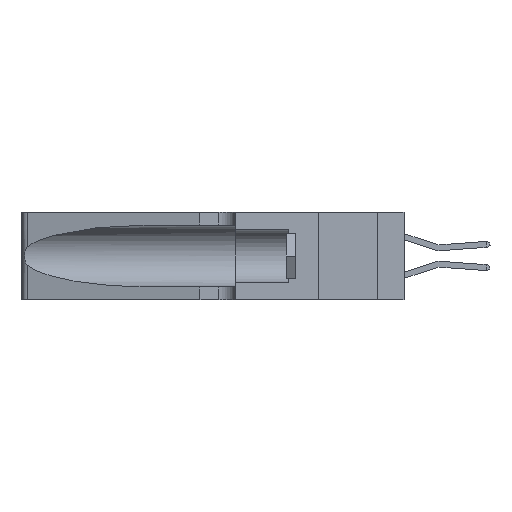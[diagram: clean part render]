
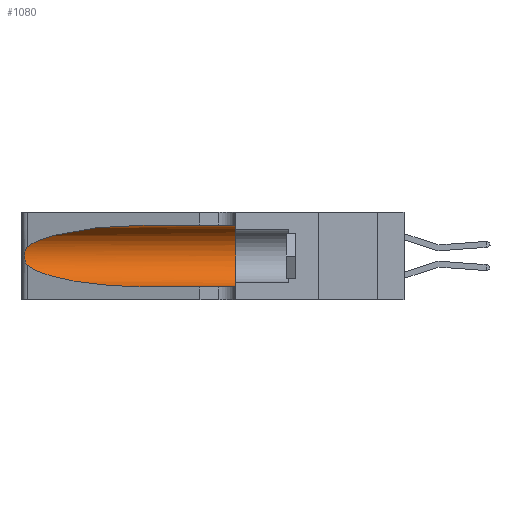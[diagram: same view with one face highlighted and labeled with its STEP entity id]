
A CAD part, left-side view. The second image highlights one B-rep face of the part: STEP entity #1080.
In plain terms, the highlighted cylindrical face has radius 3.308 mm (diameter 6.617 mm), a partial arc.
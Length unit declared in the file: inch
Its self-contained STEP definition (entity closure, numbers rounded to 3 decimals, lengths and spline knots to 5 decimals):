
#271 = CARTESIAN_POINT ( 'NONE',  ( 0.1305, 1.61858, 0.05475 ) ) ;
#1080 = ADVANCED_FACE ( 'NONE', ( #2937 ), #16985, .F. ) ;
#2819 = CARTESIAN_POINT ( 'NONE',  ( 0.25789, 1.23486, 0.15765 ) ) ;
#2937 = FACE_OUTER_BOUND ( 'NONE', #26758, .T. ) ;
#3029 = LINE ( 'NONE', #271, #32504 ) ;
#3994 = CARTESIAN_POINT ( 'NONE',  ( 0.1305, 0.72297, 0.31525 ) ) ;
#4893 = CARTESIAN_POINT ( 'NONE',  ( 0.1305, 0.72297, 0.31525 ) ) ;
#5700 = CARTESIAN_POINT ( 'NONE',  ( 0.25555, 1.22993, 0.14849 ) ) ;
#6794 = EDGE_CURVE ( 'NONE', #8950, #34060, #3029, .T. ) ;
#8090 = AXIS2_PLACEMENT_3D ( 'NONE', #16052, #35247, #18806 ) ;
#8423 = CARTESIAN_POINT ( 'NONE',  ( 0.25555, 1.22994, 0.2215 ) ) ;
#8950 = VERTEX_POINT ( 'NONE', #14795 ) ;
#9006 = CARTESIAN_POINT ( 'NONE',  ( 0.25487, 1.22718, 0.14631 ) ) ;
#9225 =( BOUNDED_CURVE ( )  B_SPLINE_CURVE ( 3, ( #4893, #10586, #32580, #16168 ),
 .UNSPECIFIED., .F., .F. ) 
 B_SPLINE_CURVE_WITH_KNOTS ( ( 4, 4 ),
 ( 1.5708, 2.84003 ),
 .UNSPECIFIED. ) 
 CURVE ( )  GEOMETRIC_REPRESENTATION_ITEM ( )  RATIONAL_B_SPLINE_CURVE ( ( 1., 0.87, 0.87, 1. ) ) 
 REPRESENTATION_ITEM ( '' )  );
#9390 = EDGE_CURVE ( 'NONE', #27486, #15746, #28443, .T. ) ;
#10586 = CARTESIAN_POINT ( 'NONE',  ( 0.18966, 0.96281, 0.31525 ) ) ;
#10595 = CARTESIAN_POINT ( 'NONE',  ( 0.18966, 0.96281, 0.05475 ) ) ;
#10683 = VECTOR ( 'NONE', #17556, 39.37008 ) ;
#11247 = CARTESIAN_POINT ( 'NONE',  ( 0.25787, 1.23484, 0.2124 ) ) ;
#12180 = ORIENTED_EDGE ( 'NONE', *, *, #18958, .T. ) ;
#14048 = CARTESIAN_POINT ( 'NONE',  ( 0.26018, 1.23835, 0.19895 ) ) ;
#14157 = CARTESIAN_POINT ( 'NONE',  ( 0.25487, 1.22718, 0.22369 ) ) ;
#14790 = CARTESIAN_POINT ( 'NONE',  ( 0.1305, 1.61858, 0.31525 ) ) ;
#14795 = CARTESIAN_POINT ( 'NONE',  ( 0.1305, 0.72297, 0.05475 ) ) ;
#15037 = CIRCLE ( 'NONE', #8090, 0.13025 ) ;
#15645 = ORIENTED_EDGE ( 'NONE', *, *, #28571, .T. ) ;
#15746 = VERTEX_POINT ( 'NONE', #9006 ) ;
#16052 = CARTESIAN_POINT ( 'NONE',  ( 0.1305, 0.35, 0.185 ) ) ;
#16168 = CARTESIAN_POINT ( 'NONE',  ( 0.25487, 1.22718, 0.22369 ) ) ;
#16812 = CARTESIAN_POINT ( 'NONE',  ( 0.26075, 1.23896, 0.178 ) ) ;
#16985 = CYLINDRICAL_SURFACE ( 'NONE', #23046, 0.13025 ) ;
#17556 = DIRECTION ( 'NONE',  ( 0., -1., 0. ) ) ;
#18230 = ORIENTED_EDGE ( 'NONE', *, *, #35185, .F. ) ;
#18806 = DIRECTION ( 'NONE',  ( 0., 0., 1. ) ) ;
#18958 = EDGE_CURVE ( 'NONE', #34624, #27486, #9225, .T. ) ;
#19579 = CARTESIAN_POINT ( 'NONE',  ( 0.25856, 1.23593, 0.16098 ) ) ;
#19929 = DIRECTION ( 'NONE',  ( 0., -1., 0. ) ) ;
#21057 = CARTESIAN_POINT ( 'NONE',  ( 0.1305, 0.35, 0.31525 ) ) ;
#22330 = CARTESIAN_POINT ( 'NONE',  ( 0.25639, 1.23186, 0.15144 ) ) ;
#23046 = AXIS2_PLACEMENT_3D ( 'NONE', #23143, #31386, #25886 ) ;
#23143 = CARTESIAN_POINT ( 'NONE',  ( 0.1305, 1.61858, 0.185 ) ) ;
#23400 = CARTESIAN_POINT ( 'NONE',  ( 0.1305, 0.35, 0.05475 ) ) ;
#23817 = ORIENTED_EDGE ( 'NONE', *, *, #28554, .F. ) ;
#24328 = CARTESIAN_POINT ( 'NONE',  ( 0.2373, 1.15595, 0.08982 ) ) ;
#24924 = VERTEX_POINT ( 'NONE', #21057 ) ;
#25091 = CARTESIAN_POINT ( 'NONE',  ( 0.25487, 1.22718, 0.14631 ) ) ;
#25798 =( BOUNDED_CURVE ( )  B_SPLINE_CURVE ( 3, ( #32465, #24328, #10595, #29829 ),
 .UNSPECIFIED., .F., .F. ) 
 B_SPLINE_CURVE_WITH_KNOTS ( ( 4, 4 ),
 ( 3.44316, 4.71239 ),
 .UNSPECIFIED. ) 
 CURVE ( )  GEOMETRIC_REPRESENTATION_ITEM ( )  RATIONAL_B_SPLINE_CURVE ( ( 1., 0.87, 0.87, 1. ) ) 
 REPRESENTATION_ITEM ( '' )  );
#25886 = DIRECTION ( 'NONE',  ( 0., 0., -1. ) ) ;
#26758 = EDGE_LOOP ( 'NONE', ( #12180, #28520, #15645, #30240, #23817, #18230 ) ) ;
#27486 = VERTEX_POINT ( 'NONE', #14157 ) ;
#27717 = CARTESIAN_POINT ( 'NONE',  ( 0.25487, 1.22718, 0.22369 ) ) ;
#28443 = B_SPLINE_CURVE_WITH_KNOTS ( 'NONE', 3,
 ( #27717, #8423, #33121, #11247, #30464, #14048, #33234, #16812, #35371, #19579, #2819, #22330, #5700, #25091 ),
 .UNSPECIFIED., .F., .F.,
 ( 4, 2, 2, 2, 2, 2, 4 ),
 ( 0., 0.00027, 0.00053, 0.00107, 0.0016, 0.00187, 0.00214 ),
 .UNSPECIFIED. ) ;
#28520 = ORIENTED_EDGE ( 'NONE', *, *, #9390, .T. ) ;
#28554 = EDGE_CURVE ( 'NONE', #24924, #34060, #15037, .T. ) ;
#28571 = EDGE_CURVE ( 'NONE', #15746, #8950, #25798, .T. ) ;
#29829 = CARTESIAN_POINT ( 'NONE',  ( 0.1305, 0.72297, 0.05475 ) ) ;
#30240 = ORIENTED_EDGE ( 'NONE', *, *, #6794, .T. ) ;
#30464 = CARTESIAN_POINT ( 'NONE',  ( 0.25854, 1.2359, 0.20912 ) ) ;
#31386 = DIRECTION ( 'NONE',  ( 0., -1., 0. ) ) ;
#32465 = CARTESIAN_POINT ( 'NONE',  ( 0.25487, 1.22718, 0.14631 ) ) ;
#32504 = VECTOR ( 'NONE', #19929, 39.37008 ) ;
#32580 = CARTESIAN_POINT ( 'NONE',  ( 0.2373, 1.15595, 0.28018 ) ) ;
#32609 = LINE ( 'NONE', #14790, #10683 ) ;
#33121 = CARTESIAN_POINT ( 'NONE',  ( 0.25639, 1.23184, 0.21858 ) ) ;
#33234 = CARTESIAN_POINT ( 'NONE',  ( 0.26075, 1.23896, 0.19203 ) ) ;
#34060 = VERTEX_POINT ( 'NONE', #23400 ) ;
#34624 = VERTEX_POINT ( 'NONE', #3994 ) ;
#35185 = EDGE_CURVE ( 'NONE', #34624, #24924, #32609, .T. ) ;
#35247 = DIRECTION ( 'NONE',  ( 0., 1., 0. ) ) ;
#35371 = CARTESIAN_POINT ( 'NONE',  ( 0.26017, 1.23833, 0.17102 ) ) ;
